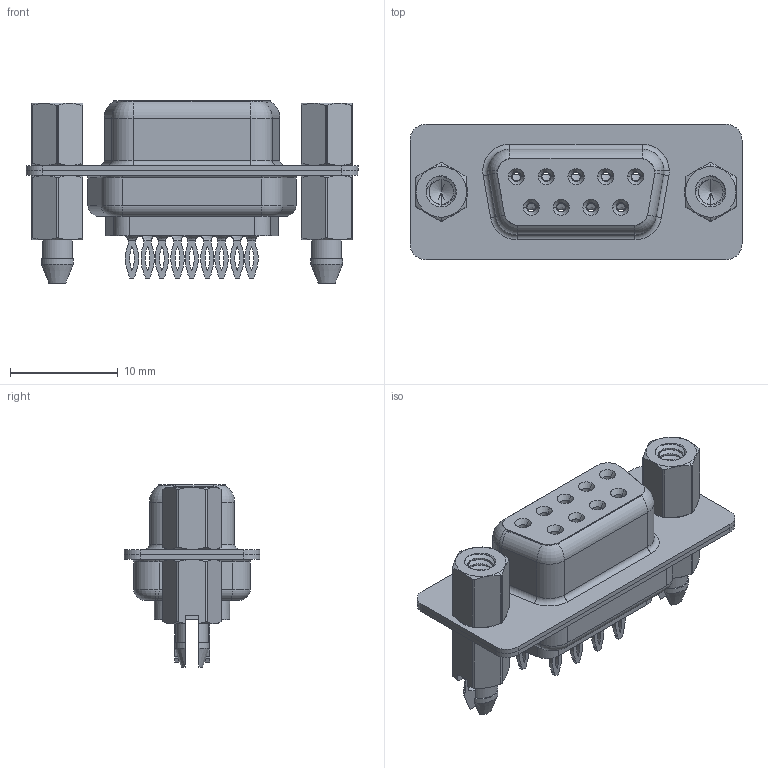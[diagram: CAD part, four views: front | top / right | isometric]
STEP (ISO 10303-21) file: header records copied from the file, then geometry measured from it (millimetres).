
FILE_DESCRIPTION (( 'STEP AP203' ), '1' );
FILE_NAME ('628-009-226-267.STEP', '2020-07-13T19:11:07', ( '' ), ( '' ), 'SwSTEP 2.0', 'SolidWorks 2020', '' );
FILE_SCHEMA (( 'CONFIG_CONTROL_DESIGN' ));
Length unit declared in the file: millimetre
Products named in the file (8): 628 Housing_09 LP; 628 4-40 Hex Standoff; 628 Contact Row 1_26L; 628 Shell Front_09 Contacts; 628 4-40 Threaded Boardlock_LP; 628-009-226-267; 628 Contact Row 2_26L; 628 Shell Rear_09 Contacts
Assembly tree (16 placements, depth 2):
  628-009-226-267
    628 Housing_09 LP
    628 Shell Front_09 Contacts
    628 Shell Rear_09 Contacts
    628 Contact Row 1_26L  x5
    628 Contact Row 2_26L  x4
    628 4-40 Hex Standoff  x2
    628 4-40 Threaded Boardlock_LP  x2
Bounding box: 30.8 x 12.6 x 16.9 mm (x, y, z)
Volume: 2084.8 mm3; surface area: 5251.4 mm2
Topology: 16 solids, 16 shells, 1388 faces, 3551 edges, 2231 vertices
Faces by surface type: cylinder 484, plane 364, bspline 234, torus 225, cone 81
Entity records: 25779 total; most frequent: CARTESIAN_POINT 9819, ORIENTED_EDGE 3192, DIRECTION 3079, EDGE_CURVE 1596, AXIS2_PLACEMENT_3D 1246, VERTEX_POINT 1008, EDGE_LOOP 712, CIRCLE 645
